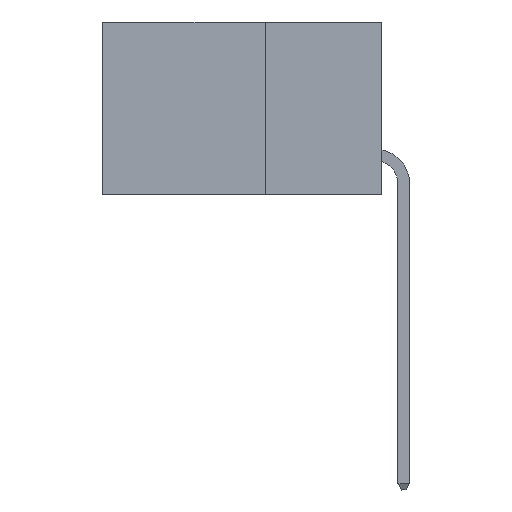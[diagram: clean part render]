
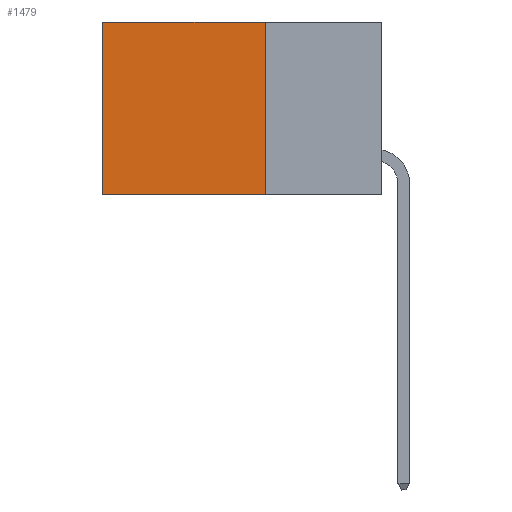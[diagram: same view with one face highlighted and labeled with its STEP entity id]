
A CAD part, left-side view. The second image highlights one B-rep face of the part: STEP entity #1479.
In plain terms, the highlighted planar face has unit normal (-1, 0, 0).
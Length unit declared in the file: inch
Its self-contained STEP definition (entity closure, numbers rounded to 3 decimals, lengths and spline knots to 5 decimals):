
#999 = DIRECTION ( 'NONE',  ( 0., 0., -1. ) ) ;
#1046 = DIRECTION ( 'NONE',  ( 0., 0., -1. ) ) ;
#1479 = ADVANCED_FACE ( 'NONE', ( #21563 ), #22912, .F. ) ;
#1832 = DIRECTION ( 'NONE',  ( 0., 1., 0. ) ) ;
#4596 = CARTESIAN_POINT ( 'NONE',  ( 0.2875, 0.25, 0. ) ) ;
#4771 = EDGE_CURVE ( 'NONE', #16751, #30129, #26773, .T. ) ;
#5518 = CARTESIAN_POINT ( 'NONE',  ( 0.2875, 0.6, 0. ) ) ;
#7126 = DIRECTION ( 'NONE',  ( 0., 1., 0. ) ) ;
#9268 = ORIENTED_EDGE ( 'NONE', *, *, #4771, .T. ) ;
#10448 = CARTESIAN_POINT ( 'NONE',  ( 0.2875, 0.6, 0. ) ) ;
#11152 = ORIENTED_EDGE ( 'NONE', *, *, #12559, .F. ) ;
#11985 = ORIENTED_EDGE ( 'NONE', *, *, #18097, .T. ) ;
#12559 = EDGE_CURVE ( 'NONE', #16751, #27421, #19489, .T. ) ;
#14443 = CARTESIAN_POINT ( 'NONE',  ( 0.2875, 0.25, 0. ) ) ;
#14475 = AXIS2_PLACEMENT_3D ( 'NONE', #14443, #14737, #16971 ) ;
#14737 = DIRECTION ( 'NONE',  ( 1., 0., 0. ) ) ;
#16130 = LINE ( 'NONE', #10448, #19599 ) ;
#16751 = VERTEX_POINT ( 'NONE', #4596 ) ;
#16971 = DIRECTION ( 'NONE',  ( 0., 0., -1. ) ) ;
#17114 = VERTEX_POINT ( 'NONE', #30840 ) ;
#18097 = EDGE_CURVE ( 'NONE', #30129, #17114, #16130, .T. ) ;
#18528 = ORIENTED_EDGE ( 'NONE', *, *, #28310, .F. ) ;
#19032 = CARTESIAN_POINT ( 'NONE',  ( 0.2875, 0.25, -0.37 ) ) ;
#19489 = LINE ( 'NONE', #23041, #26004 ) ;
#19599 = VECTOR ( 'NONE', #999, 39.37008 ) ;
#20248 = CARTESIAN_POINT ( 'NONE',  ( 0.2875, 0.25, -0.37 ) ) ;
#21563 = FACE_OUTER_BOUND ( 'NONE', #24215, .T. ) ;
#22912 = PLANE ( 'NONE',  #14475 ) ;
#23041 = CARTESIAN_POINT ( 'NONE',  ( 0.2875, 0.25, 0. ) ) ;
#23820 = CARTESIAN_POINT ( 'NONE',  ( 0.2875, 0.25, 0. ) ) ;
#24215 = EDGE_LOOP ( 'NONE', ( #11985, #18528, #11152, #9268 ) ) ;
#25222 = LINE ( 'NONE', #19032, #27131 ) ;
#26004 = VECTOR ( 'NONE', #1046, 39.37008 ) ;
#26773 = LINE ( 'NONE', #23820, #30990 ) ;
#27131 = VECTOR ( 'NONE', #7126, 39.37008 ) ;
#27421 = VERTEX_POINT ( 'NONE', #20248 ) ;
#28310 = EDGE_CURVE ( 'NONE', #27421, #17114, #25222, .T. ) ;
#30129 = VERTEX_POINT ( 'NONE', #5518 ) ;
#30840 = CARTESIAN_POINT ( 'NONE',  ( 0.2875, 0.6, -0.37 ) ) ;
#30990 = VECTOR ( 'NONE', #1832, 39.37008 ) ;
